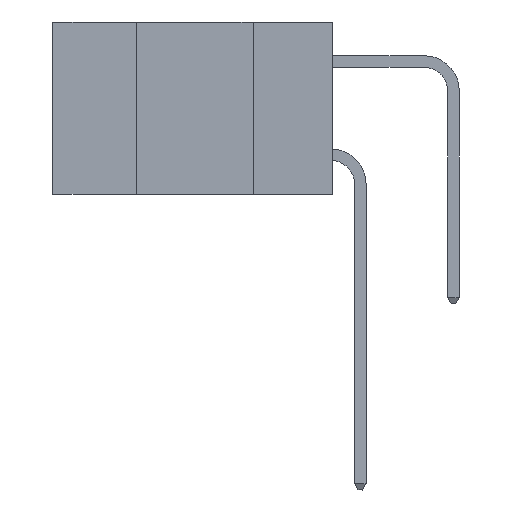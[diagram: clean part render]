
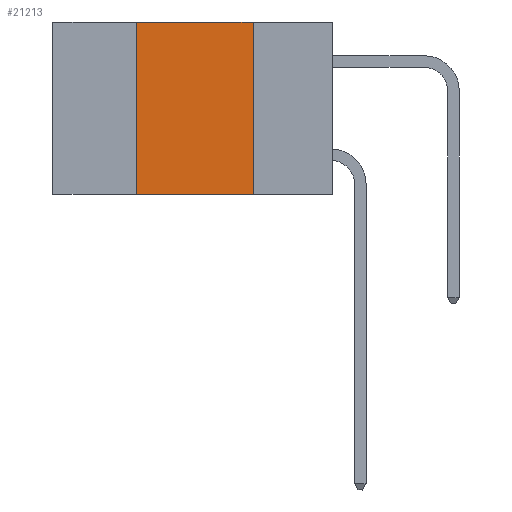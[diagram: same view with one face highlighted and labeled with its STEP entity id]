
A CAD part, left-side view. The second image highlights one B-rep face of the part: STEP entity #21213.
In plain terms, the highlighted planar face has unit normal (-1, 0, 0).
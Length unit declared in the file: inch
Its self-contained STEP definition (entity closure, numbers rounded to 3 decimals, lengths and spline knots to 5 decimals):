
#119 = VECTOR ( 'NONE', #4619, 39.37008 ) ;
#570 = PLANE ( 'NONE',  #7199 ) ;
#2339 = CARTESIAN_POINT ( 'NONE',  ( 0., 0.6, -0.37 ) ) ;
#4009 = VERTEX_POINT ( 'NONE', #18626 ) ;
#4329 = CARTESIAN_POINT ( 'NONE',  ( 0., 0.17, 0. ) ) ;
#4619 = DIRECTION ( 'NONE',  ( 0., -1., 0. ) ) ;
#4732 = VERTEX_POINT ( 'NONE', #7490 ) ;
#6948 = DIRECTION ( 'NONE',  ( 0., -1., 0. ) ) ;
#7199 = AXIS2_PLACEMENT_3D ( 'NONE', #11447, #27053, #16486 ) ;
#7490 = CARTESIAN_POINT ( 'NONE',  ( 0., 0.42, -0.37 ) ) ;
#8965 = EDGE_CURVE ( 'NONE', #4732, #21771, #10623, .T. ) ;
#8968 = CARTESIAN_POINT ( 'NONE',  ( 0., 0.17, -0.37 ) ) ;
#9731 = VECTOR ( 'NONE', #12851, 39.37008 ) ;
#10021 = DIRECTION ( 'NONE',  ( 0., 0., 1. ) ) ;
#10623 = LINE ( 'NONE', #2339, #119 ) ;
#11447 = CARTESIAN_POINT ( 'NONE',  ( 0., 0.6, 0. ) ) ;
#11645 = EDGE_LOOP ( 'NONE', ( #16878, #22772, #21755, #24541 ) ) ;
#11657 = CARTESIAN_POINT ( 'NONE',  ( 0., 0.6, 0. ) ) ;
#12851 = DIRECTION ( 'NONE',  ( 0., 0., -1. ) ) ;
#13450 = LINE ( 'NONE', #4329, #9731 ) ;
#13818 = CARTESIAN_POINT ( 'NONE',  ( 0., 0.42, 0. ) ) ;
#15108 = LINE ( 'NONE', #11657, #16084 ) ;
#15287 = VECTOR ( 'NONE', #10021, 39.37008 ) ;
#15661 = EDGE_CURVE ( 'NONE', #4732, #25778, #26724, .T. ) ;
#16084 = VECTOR ( 'NONE', #6948, 39.37008 ) ;
#16486 = DIRECTION ( 'NONE',  ( 0., 0., -1. ) ) ;
#16878 = ORIENTED_EDGE ( 'NONE', *, *, #23737, .F. ) ;
#17139 = CARTESIAN_POINT ( 'NONE',  ( 0., 0.42, 0. ) ) ;
#18626 = CARTESIAN_POINT ( 'NONE',  ( 0., 0.17, 0. ) ) ;
#18832 = EDGE_CURVE ( 'NONE', #25778, #4009, #15108, .T. ) ;
#21213 = ADVANCED_FACE ( 'NONE', ( #25381 ), #570, .F. ) ;
#21755 = ORIENTED_EDGE ( 'NONE', *, *, #15661, .F. ) ;
#21771 = VERTEX_POINT ( 'NONE', #8968 ) ;
#22772 = ORIENTED_EDGE ( 'NONE', *, *, #18832, .F. ) ;
#23737 = EDGE_CURVE ( 'NONE', #4009, #21771, #13450, .T. ) ;
#24541 = ORIENTED_EDGE ( 'NONE', *, *, #8965, .T. ) ;
#25381 = FACE_OUTER_BOUND ( 'NONE', #11645, .T. ) ;
#25778 = VERTEX_POINT ( 'NONE', #17139 ) ;
#26724 = LINE ( 'NONE', #13818, #15287 ) ;
#27053 = DIRECTION ( 'NONE',  ( 1., 0., 0. ) ) ;
